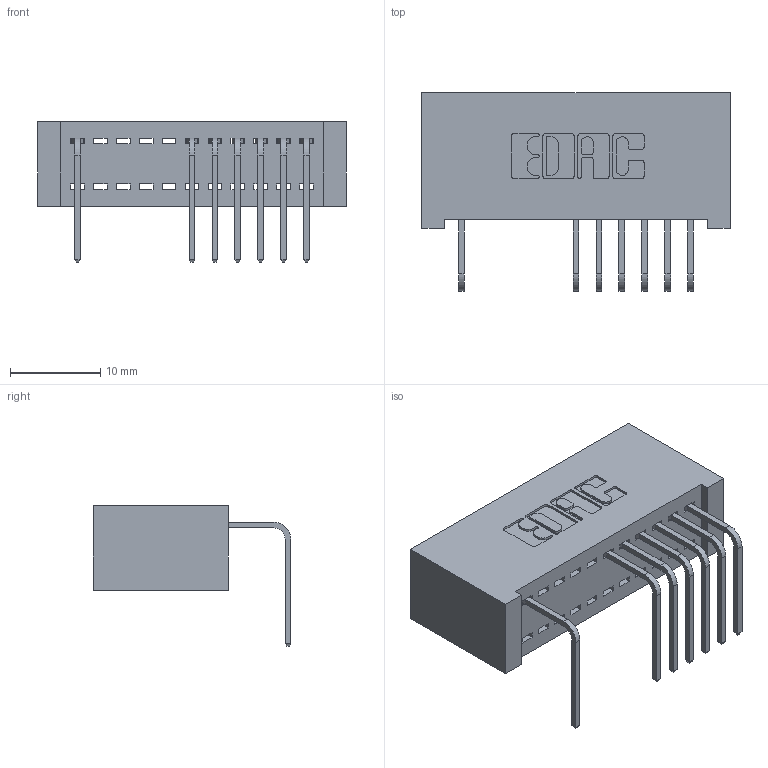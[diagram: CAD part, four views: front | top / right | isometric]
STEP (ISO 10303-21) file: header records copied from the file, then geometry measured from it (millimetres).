
FILE_DESCRIPTION (( 'STEP AP203' ), '1' );
FILE_NAME ('342-011-558-101.STEP', '2018-08-10T14:39:05', ( '' ), ( '' ), 'SwSTEP 2.0', 'SolidWorks 2016', '' );
FILE_SCHEMA (( 'CONFIG_CONTROL_DESIGN' ));
Length unit declared in the file: inch
Products named in the file (3): 342 Part_Lugless; 345-292-001_558 Tail - 2; 342-011-558-101
Assembly tree (8 placements, depth 2):
  342-011-558-101
    342 Part_Lugless
    345-292-001_558 Tail - 2  x7
Bounding box: 34.19 x 21.91 x 15.62 mm (x, y, z)
Volume: 3270 mm3; surface area: 4441.7 mm2
Topology: 8 solids, 8 shells, 570 faces, 1717 edges, 1134 vertices
Faces by surface type: plane 418, cylinder 152
Entity records: 10281 total; most frequent: CARTESIAN_POINT 1803, ORIENTED_EDGE 1754, DIRECTION 1571, EDGE_CURVE 877, VECTOR 757, LINE 757, VERTEX_POINT 582, AXIS2_PLACEMENT_3D 407
